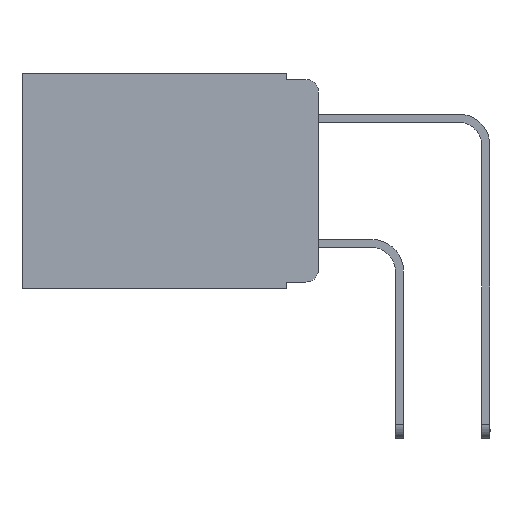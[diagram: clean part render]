
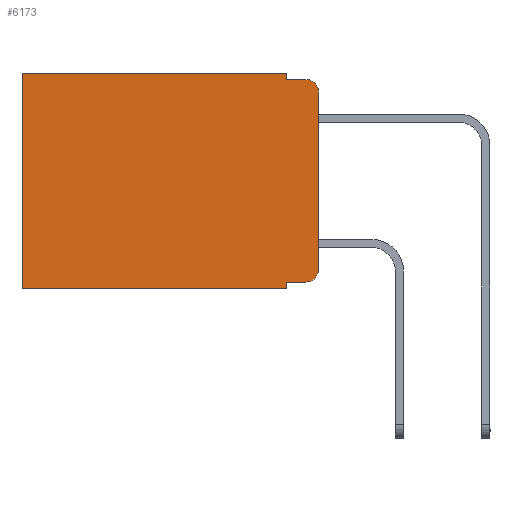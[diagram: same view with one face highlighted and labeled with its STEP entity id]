
A CAD part, left-side view. The second image highlights one B-rep face of the part: STEP entity #6173.
In plain terms, the highlighted planar face has unit normal (-1, 0, 0).
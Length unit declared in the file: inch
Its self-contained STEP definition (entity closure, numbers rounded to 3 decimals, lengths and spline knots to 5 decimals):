
#148 = DIRECTION ( 'NONE',  ( 0., 0., -1. ) ) ;
#463 = VERTEX_POINT ( 'NONE', #8303 ) ;
#529 = CARTESIAN_POINT ( 'NONE',  ( 0.298, 0.02, -0.333 ) ) ;
#844 = AXIS2_PLACEMENT_3D ( 'NONE', #9778, #4685, #3757 ) ;
#985 = LINE ( 'NONE', #8561, #2308 ) ;
#1005 = DIRECTION ( 'NONE',  ( 0., -1., 0. ) ) ;
#1300 = DIRECTION ( 'NONE',  ( 0., -1., 0. ) ) ;
#1362 = EDGE_CURVE ( 'NONE', #4277, #463, #7944, .T. ) ;
#1375 = ORIENTED_EDGE ( 'NONE', *, *, #1816, .T. ) ;
#1714 = CARTESIAN_POINT ( 'NONE',  ( 0.298, 0.051, 0. ) ) ;
#1815 = VECTOR ( 'NONE', #1868, 39.37008 ) ;
#1816 = EDGE_CURVE ( 'NONE', #3717, #8898, #4192, .T. ) ;
#1868 = DIRECTION ( 'NONE',  ( 0., 0., -1. ) ) ;
#2308 = VECTOR ( 'NONE', #1005, 39.37008 ) ;
#2342 = DIRECTION ( 'NONE',  ( 0., 0., -1. ) ) ;
#2362 = ORIENTED_EDGE ( 'NONE', *, *, #7422, .F. ) ;
#2483 = CARTESIAN_POINT ( 'NONE',  ( 0.298, 0., -0.03 ) ) ;
#2678 = CARTESIAN_POINT ( 'NONE',  ( 0.298, 0.051, -0.333 ) ) ;
#2760 = EDGE_CURVE ( 'NONE', #3728, #5482, #6053, .T. ) ;
#2891 = AXIS2_PLACEMENT_3D ( 'NONE', #7076, #8840, #3788 ) ;
#3004 = PLANE ( 'NONE',  #844 ) ;
#3059 = DIRECTION ( 'NONE',  ( -1., 0., 0. ) ) ;
#3141 = ORIENTED_EDGE ( 'NONE', *, *, #7644, .T. ) ;
#3159 = EDGE_CURVE ( 'NONE', #3717, #6562, #4053, .T. ) ;
#3362 = VECTOR ( 'NONE', #10784, 39.37008 ) ;
#3463 = ORIENTED_EDGE ( 'NONE', *, *, #7830, .F. ) ;
#3717 = VERTEX_POINT ( 'NONE', #2678 ) ;
#3728 = VERTEX_POINT ( 'NONE', #1714 ) ;
#3757 = DIRECTION ( 'NONE',  ( 0., 0., -1. ) ) ;
#3781 = VECTOR ( 'NONE', #4080, 39.37008 ) ;
#3788 = DIRECTION ( 'NONE',  ( 0., 0., -1. ) ) ;
#3816 = CARTESIAN_POINT ( 'NONE',  ( 0.298, 0.02, -0.03 ) ) ;
#3954 = CARTESIAN_POINT ( 'NONE',  ( 0.298, 0., 0. ) ) ;
#4053 = LINE ( 'NONE', #8673, #1815 ) ;
#4080 = DIRECTION ( 'NONE',  ( 0., 0., -1. ) ) ;
#4167 = AXIS2_PLACEMENT_3D ( 'NONE', #3816, #3059, #9023 ) ;
#4192 = LINE ( 'NONE', #4731, #10835 ) ;
#4202 = CARTESIAN_POINT ( 'NONE',  ( 0.298, 0.051, -0.01 ) ) ;
#4241 = VERTEX_POINT ( 'NONE', #5051 ) ;
#4277 = VERTEX_POINT ( 'NONE', #2483 ) ;
#4390 = CARTESIAN_POINT ( 'NONE',  ( 0.298, 0.473, 0. ) ) ;
#4540 = LINE ( 'NONE', #10525, #9875 ) ;
#4685 = DIRECTION ( 'NONE',  ( 1., 0., 0. ) ) ;
#4731 = CARTESIAN_POINT ( 'NONE',  ( 0.298, 0.051, -0.333 ) ) ;
#4837 = EDGE_CURVE ( 'NONE', #10785, #6696, #5948, .T. ) ;
#5051 = CARTESIAN_POINT ( 'NONE',  ( 0.298, 0.02, -0.01 ) ) ;
#5482 = VERTEX_POINT ( 'NONE', #4202 ) ;
#5522 = CIRCLE ( 'NONE', #2891, 0.02 ) ;
#5629 = EDGE_CURVE ( 'NONE', #8898, #463, #5522, .T. ) ;
#5688 = CARTESIAN_POINT ( 'NONE',  ( 0.298, 0.051, 0. ) ) ;
#5887 = ORIENTED_EDGE ( 'NONE', *, *, #3159, .F. ) ;
#5948 = LINE ( 'NONE', #4390, #10844 ) ;
#6053 = LINE ( 'NONE', #5688, #3781 ) ;
#6173 = ADVANCED_FACE ( 'NONE', ( #6460 ), #3004, .F. ) ;
#6460 = FACE_OUTER_BOUND ( 'NONE', #7297, .T. ) ;
#6562 = VERTEX_POINT ( 'NONE', #10148 ) ;
#6652 = CIRCLE ( 'NONE', #4167, 0.02 ) ;
#6696 = VERTEX_POINT ( 'NONE', #10467 ) ;
#6736 = ORIENTED_EDGE ( 'NONE', *, *, #4837, .T. ) ;
#7054 = DIRECTION ( 'NONE',  ( 0., 1., 0. ) ) ;
#7076 = CARTESIAN_POINT ( 'NONE',  ( 0.298, 0.02, -0.313 ) ) ;
#7287 = ORIENTED_EDGE ( 'NONE', *, *, #9317, .T. ) ;
#7297 = EDGE_LOOP ( 'NONE', ( #10474, #7287, #3463, #8428, #3141, #6736, #2362, #5887, #1375, #10624 ) ) ;
#7422 = EDGE_CURVE ( 'NONE', #6562, #6696, #4540, .T. ) ;
#7644 = EDGE_CURVE ( 'NONE', #3728, #10785, #7881, .T. ) ;
#7830 = EDGE_CURVE ( 'NONE', #5482, #4241, #985, .T. ) ;
#7881 = LINE ( 'NONE', #3954, #3362 ) ;
#7944 = LINE ( 'NONE', #8161, #10584 ) ;
#8161 = CARTESIAN_POINT ( 'NONE',  ( 0.298, 0., 0. ) ) ;
#8303 = CARTESIAN_POINT ( 'NONE',  ( 0.298, 0., -0.313 ) ) ;
#8428 = ORIENTED_EDGE ( 'NONE', *, *, #2760, .F. ) ;
#8561 = CARTESIAN_POINT ( 'NONE',  ( 0.298, 0.051, -0.01 ) ) ;
#8623 = CARTESIAN_POINT ( 'NONE',  ( 0.298, 0.473, 0. ) ) ;
#8673 = CARTESIAN_POINT ( 'NONE',  ( 0.298, 0.051, 0. ) ) ;
#8840 = DIRECTION ( 'NONE',  ( -1., 0., 0. ) ) ;
#8898 = VERTEX_POINT ( 'NONE', #529 ) ;
#9023 = DIRECTION ( 'NONE',  ( 0., 0., -1. ) ) ;
#9317 = EDGE_CURVE ( 'NONE', #4277, #4241, #6652, .T. ) ;
#9778 = CARTESIAN_POINT ( 'NONE',  ( 0.298, 0., 0. ) ) ;
#9875 = VECTOR ( 'NONE', #7054, 39.37008 ) ;
#10148 = CARTESIAN_POINT ( 'NONE',  ( 0.298, 0.051, -0.343 ) ) ;
#10467 = CARTESIAN_POINT ( 'NONE',  ( 0.298, 0.473, -0.343 ) ) ;
#10474 = ORIENTED_EDGE ( 'NONE', *, *, #1362, .F. ) ;
#10525 = CARTESIAN_POINT ( 'NONE',  ( 0.298, 0., -0.343 ) ) ;
#10584 = VECTOR ( 'NONE', #2342, 39.37008 ) ;
#10624 = ORIENTED_EDGE ( 'NONE', *, *, #5629, .T. ) ;
#10784 = DIRECTION ( 'NONE',  ( 0., 1., 0. ) ) ;
#10785 = VERTEX_POINT ( 'NONE', #8623 ) ;
#10835 = VECTOR ( 'NONE', #1300, 39.37008 ) ;
#10844 = VECTOR ( 'NONE', #148, 39.37008 ) ;
